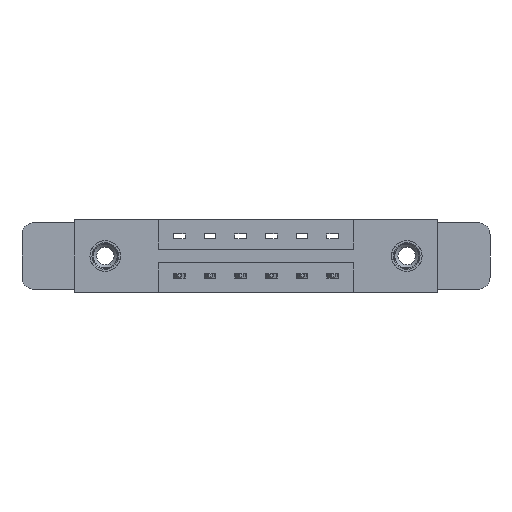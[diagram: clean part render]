
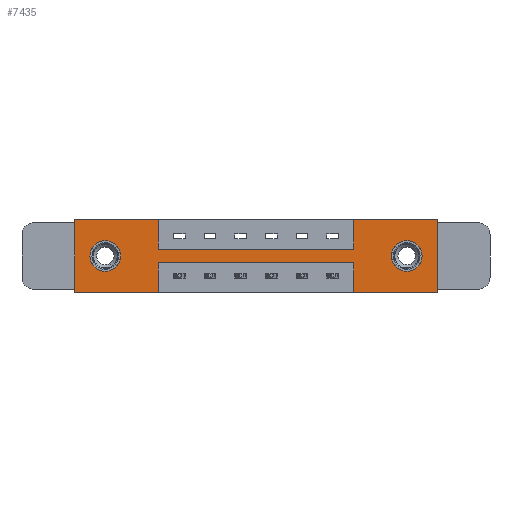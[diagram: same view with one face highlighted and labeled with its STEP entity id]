
A CAD part, front view. The second image highlights one B-rep face of the part: STEP entity #7435.
In plain terms, the highlighted planar face has unit normal (0, -1, 0).
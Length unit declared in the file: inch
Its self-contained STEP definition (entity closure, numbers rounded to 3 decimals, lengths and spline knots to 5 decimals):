
#233 = EDGE_CURVE ( 'NONE', #6314, #7946, #9109, .T. ) ;
#349 = FACE_BOUND ( 'NONE', #4689, .T. ) ;
#622 = EDGE_CURVE ( 'NONE', #1587, #2088, #11667, .T. ) ;
#685 = VECTOR ( 'NONE', #7072, 39.37008 ) ;
#703 = CARTESIAN_POINT ( 'NONE',  ( 1.417, 0., -0.37 ) ) ;
#887 = VECTOR ( 'NONE', #5245, 39.37008 ) ;
#939 = EDGE_CURVE ( 'NONE', #9607, #5878, #6537, .T. ) ;
#959 = AXIS2_PLACEMENT_3D ( 'NONE', #9314, #11021, #7533 ) ;
#1142 = EDGE_CURVE ( 'NONE', #8023, #9607, #3968, .T. ) ;
#1169 = PLANE ( 'NONE',  #5364 ) ;
#1181 = CARTESIAN_POINT ( 'NONE',  ( 1.417, 0., -0.22 ) ) ;
#1190 = EDGE_CURVE ( 'NONE', #3699, #6756, #9629, .T. ) ;
#1209 = CARTESIAN_POINT ( 'NONE',  ( 0.425, 0., 0. ) ) ;
#1222 = CARTESIAN_POINT ( 'NONE',  ( 1.687, 0., -0.263 ) ) ;
#1284 = ORIENTED_EDGE ( 'NONE', *, *, #1142, .F. ) ;
#1312 = ORIENTED_EDGE ( 'NONE', *, *, #2669, .F. ) ;
#1545 = CARTESIAN_POINT ( 'NONE',  ( 1.687, 0., -0.185 ) ) ;
#1587 = VERTEX_POINT ( 'NONE', #1774 ) ;
#1593 = DIRECTION ( 'NONE',  ( 0., 1., 0. ) ) ;
#1663 = CARTESIAN_POINT ( 'NONE',  ( 0., 0., -0.37 ) ) ;
#1678 = DIRECTION ( 'NONE',  ( 1., 0., 0. ) ) ;
#1774 = CARTESIAN_POINT ( 'NONE',  ( 0.425, 0., -0.37 ) ) ;
#1783 = EDGE_CURVE ( 'NONE', #6987, #1587, #10924, .T. ) ;
#1792 = CARTESIAN_POINT ( 'NONE',  ( 0.425, 0., -0.15 ) ) ;
#1838 = VECTOR ( 'NONE', #11322, 39.37008 ) ;
#1839 = ORIENTED_EDGE ( 'NONE', *, *, #5747, .F. ) ;
#1851 = ORIENTED_EDGE ( 'NONE', *, *, #1783, .F. ) ;
#2088 = VERTEX_POINT ( 'NONE', #2337 ) ;
#2230 = LINE ( 'NONE', #9575, #11634 ) ;
#2337 = CARTESIAN_POINT ( 'NONE',  ( 0., 0., -0.37 ) ) ;
#2480 = CIRCLE ( 'NONE', #959, 0.078 ) ;
#2516 = VECTOR ( 'NONE', #3381, 39.37008 ) ;
#2639 = CARTESIAN_POINT ( 'NONE',  ( 1.417, 0., 0. ) ) ;
#2669 = EDGE_CURVE ( 'NONE', #6756, #6987, #8936, .T. ) ;
#3036 = ORIENTED_EDGE ( 'NONE', *, *, #1190, .F. ) ;
#3053 = DIRECTION ( 'NONE',  ( 0., 0., -1. ) ) ;
#3109 = ORIENTED_EDGE ( 'NONE', *, *, #622, .F. ) ;
#3381 = DIRECTION ( 'NONE',  ( -1., 0., 0. ) ) ;
#3460 = ORIENTED_EDGE ( 'NONE', *, *, #10895, .T. ) ;
#3699 = VERTEX_POINT ( 'NONE', #703 ) ;
#3825 = CARTESIAN_POINT ( 'NONE',  ( 0., 0., -0.37 ) ) ;
#3832 = LINE ( 'NONE', #1209, #11643 ) ;
#3951 = EDGE_CURVE ( 'NONE', #9813, #4037, #7751, .T. ) ;
#3968 = LINE ( 'NONE', #2639, #10346 ) ;
#4018 = VERTEX_POINT ( 'NONE', #10889 ) ;
#4037 = VERTEX_POINT ( 'NONE', #7592 ) ;
#4039 = ORIENTED_EDGE ( 'NONE', *, *, #3951, .T. ) ;
#4107 = CARTESIAN_POINT ( 'NONE',  ( 0.425, 0., -0.15 ) ) ;
#4321 = CARTESIAN_POINT ( 'NONE',  ( 0., 0., 0. ) ) ;
#4408 = CARTESIAN_POINT ( 'NONE',  ( 1.842, 0., -0.37 ) ) ;
#4410 = AXIS2_PLACEMENT_3D ( 'NONE', #7383, #9235, #9195 ) ;
#4414 = VECTOR ( 'NONE', #10772, 39.37008 ) ;
#4535 = VECTOR ( 'NONE', #8015, 39.37008 ) ;
#4689 = EDGE_LOOP ( 'NONE', ( #3460, #4899 ) ) ;
#4715 = LINE ( 'NONE', #4107, #1838 ) ;
#4820 = EDGE_CURVE ( 'NONE', #4037, #9813, #10359, .T. ) ;
#4899 = ORIENTED_EDGE ( 'NONE', *, *, #10798, .T. ) ;
#5033 = CIRCLE ( 'NONE', #4410, 0.078 ) ;
#5167 = EDGE_LOOP ( 'NONE', ( #8041, #4039 ) ) ;
#5245 = DIRECTION ( 'NONE',  ( -1., 0., 0. ) ) ;
#5364 = AXIS2_PLACEMENT_3D ( 'NONE', #3825, #7549, #3053 ) ;
#5638 = EDGE_CURVE ( 'NONE', #7946, #9088, #3832, .T. ) ;
#5685 = VECTOR ( 'NONE', #7642, 39.37008 ) ;
#5721 = ORIENTED_EDGE ( 'NONE', *, *, #233, .F. ) ;
#5747 = EDGE_CURVE ( 'NONE', #5878, #5790, #6969, .T. ) ;
#5790 = VERTEX_POINT ( 'NONE', #4408 ) ;
#5878 = VERTEX_POINT ( 'NONE', #11553 ) ;
#5973 = DIRECTION ( 'NONE',  ( 0., 0., 1. ) ) ;
#6244 = AXIS2_PLACEMENT_3D ( 'NONE', #1545, #1593, #7148 ) ;
#6254 = CARTESIAN_POINT ( 'NONE',  ( 1.417, 0., -0.37 ) ) ;
#6314 = VERTEX_POINT ( 'NONE', #6942 ) ;
#6428 = EDGE_CURVE ( 'NONE', #2088, #6314, #2230, .T. ) ;
#6438 = CARTESIAN_POINT ( 'NONE',  ( 0.155, 0., -0.263 ) ) ;
#6537 = LINE ( 'NONE', #4321, #685 ) ;
#6756 = VERTEX_POINT ( 'NONE', #1181 ) ;
#6807 = VECTOR ( 'NONE', #6834, 39.37008 ) ;
#6834 = DIRECTION ( 'NONE',  ( 0., 0., -1. ) ) ;
#6942 = CARTESIAN_POINT ( 'NONE',  ( 0., 0., 0. ) ) ;
#6969 = LINE ( 'NONE', #11348, #6807 ) ;
#6987 = VERTEX_POINT ( 'NONE', #9720 ) ;
#7007 = CARTESIAN_POINT ( 'NONE',  ( 0.425, 0., 0. ) ) ;
#7072 = DIRECTION ( 'NONE',  ( 1., 0., 0. ) ) ;
#7148 = DIRECTION ( 'NONE',  ( 0., 0., -1. ) ) ;
#7383 = CARTESIAN_POINT ( 'NONE',  ( 0.155, 0., -0.185 ) ) ;
#7435 = ADVANCED_FACE ( 'NONE', ( #7763, #349, #9175 ), #1169, .T. ) ;
#7499 = ORIENTED_EDGE ( 'NONE', *, *, #6428, .F. ) ;
#7533 = DIRECTION ( 'NONE',  ( 0., 0., 1. ) ) ;
#7549 = DIRECTION ( 'NONE',  ( 0., -1., 0. ) ) ;
#7592 = CARTESIAN_POINT ( 'NONE',  ( 1.687, 0., -0.107 ) ) ;
#7606 = CARTESIAN_POINT ( 'NONE',  ( 0.425, 0., -0.37 ) ) ;
#7642 = DIRECTION ( 'NONE',  ( 0., 0., -1. ) ) ;
#7751 = CIRCLE ( 'NONE', #6244, 0.078 ) ;
#7763 = FACE_BOUND ( 'NONE', #5167, .T. ) ;
#7775 = AXIS2_PLACEMENT_3D ( 'NONE', #11635, #8743, #11463 ) ;
#7833 = VECTOR ( 'NONE', #1678, 39.37008 ) ;
#7910 = CARTESIAN_POINT ( 'NONE',  ( 1.417, 0., -0.15 ) ) ;
#7946 = VERTEX_POINT ( 'NONE', #7007 ) ;
#8015 = DIRECTION ( 'NONE',  ( 0., 0., 1. ) ) ;
#8023 = VERTEX_POINT ( 'NONE', #7910 ) ;
#8041 = ORIENTED_EDGE ( 'NONE', *, *, #4820, .T. ) ;
#8042 = ORIENTED_EDGE ( 'NONE', *, *, #8817, .F. ) ;
#8087 = VERTEX_POINT ( 'NONE', #6438 ) ;
#8252 = CARTESIAN_POINT ( 'NONE',  ( 1.417, 0., 0. ) ) ;
#8424 = ORIENTED_EDGE ( 'NONE', *, *, #10005, .F. ) ;
#8743 = DIRECTION ( 'NONE',  ( 0., 1., 0. ) ) ;
#8817 = EDGE_CURVE ( 'NONE', #5790, #3699, #11713, .T. ) ;
#8936 = LINE ( 'NONE', #11423, #2516 ) ;
#9088 = VERTEX_POINT ( 'NONE', #1792 ) ;
#9109 = LINE ( 'NONE', #9860, #7833 ) ;
#9175 = FACE_OUTER_BOUND ( 'NONE', #10638, .T. ) ;
#9195 = DIRECTION ( 'NONE',  ( 0., 0., 1. ) ) ;
#9235 = DIRECTION ( 'NONE',  ( 0., 1., 0. ) ) ;
#9314 = CARTESIAN_POINT ( 'NONE',  ( 0.155, 0., -0.185 ) ) ;
#9575 = CARTESIAN_POINT ( 'NONE',  ( 0., 0., 0. ) ) ;
#9607 = VERTEX_POINT ( 'NONE', #8252 ) ;
#9629 = LINE ( 'NONE', #6254, #4535 ) ;
#9674 = CARTESIAN_POINT ( 'NONE',  ( 0., 0., -0.37 ) ) ;
#9720 = CARTESIAN_POINT ( 'NONE',  ( 0.425, 0., -0.22 ) ) ;
#9813 = VERTEX_POINT ( 'NONE', #1222 ) ;
#9860 = CARTESIAN_POINT ( 'NONE',  ( 0., 0., 0. ) ) ;
#10005 = EDGE_CURVE ( 'NONE', #9088, #8023, #4715, .T. ) ;
#10346 = VECTOR ( 'NONE', #10775, 39.37008 ) ;
#10359 = CIRCLE ( 'NONE', #7775, 0.078 ) ;
#10417 = ORIENTED_EDGE ( 'NONE', *, *, #5638, .F. ) ;
#10473 = DIRECTION ( 'NONE',  ( 0., 0., -1. ) ) ;
#10638 = EDGE_LOOP ( 'NONE', ( #1851, #1312, #3036, #8042, #1839, #11315, #1284, #8424, #10417, #5721, #7499, #3109 ) ) ;
#10772 = DIRECTION ( 'NONE',  ( -1., 0., 0. ) ) ;
#10775 = DIRECTION ( 'NONE',  ( 0., 0., 1. ) ) ;
#10798 = EDGE_CURVE ( 'NONE', #8087, #4018, #5033, .T. ) ;
#10889 = CARTESIAN_POINT ( 'NONE',  ( 0.155, 0., -0.107 ) ) ;
#10895 = EDGE_CURVE ( 'NONE', #4018, #8087, #2480, .T. ) ;
#10924 = LINE ( 'NONE', #7606, #5685 ) ;
#11021 = DIRECTION ( 'NONE',  ( 0., 1., 0. ) ) ;
#11315 = ORIENTED_EDGE ( 'NONE', *, *, #939, .F. ) ;
#11322 = DIRECTION ( 'NONE',  ( 1., 0., 0. ) ) ;
#11348 = CARTESIAN_POINT ( 'NONE',  ( 1.842, 0., 0. ) ) ;
#11423 = CARTESIAN_POINT ( 'NONE',  ( 0.425, 0., -0.22 ) ) ;
#11463 = DIRECTION ( 'NONE',  ( 0., 0., -1. ) ) ;
#11553 = CARTESIAN_POINT ( 'NONE',  ( 1.842, 0., 0. ) ) ;
#11634 = VECTOR ( 'NONE', #5973, 39.37008 ) ;
#11635 = CARTESIAN_POINT ( 'NONE',  ( 1.687, 0., -0.185 ) ) ;
#11643 = VECTOR ( 'NONE', #10473, 39.37008 ) ;
#11667 = LINE ( 'NONE', #1663, #4414 ) ;
#11713 = LINE ( 'NONE', #9674, #887 ) ;
